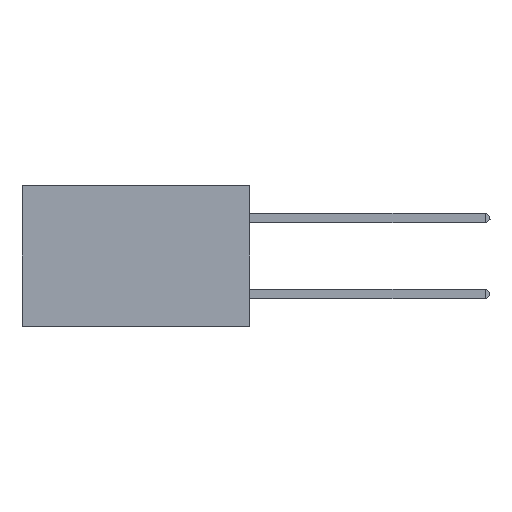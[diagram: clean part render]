
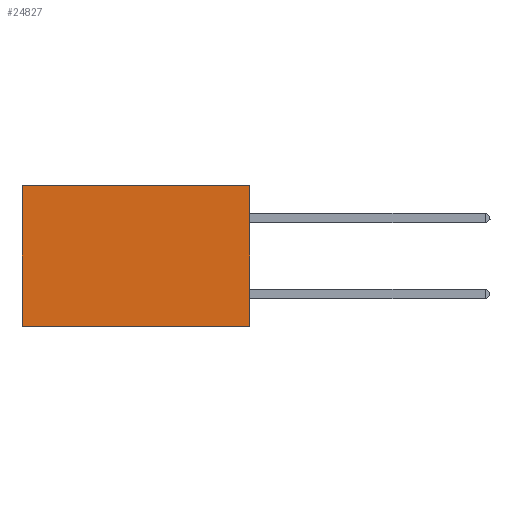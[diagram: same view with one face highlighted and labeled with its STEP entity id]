
A CAD part, left-side view. The second image highlights one B-rep face of the part: STEP entity #24827.
In plain terms, the highlighted planar face has unit normal (-1, 0, 0).
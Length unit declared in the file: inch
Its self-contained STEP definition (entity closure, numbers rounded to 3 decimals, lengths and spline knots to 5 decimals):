
#881 = CARTESIAN_POINT ( 'NONE',  ( 0.2875, 0., -0.37 ) ) ;
#1184 = EDGE_CURVE ( 'NONE', #18749, #23973, #15874, .T. ) ;
#1930 = EDGE_CURVE ( 'NONE', #21699, #4590, #20369, .T. ) ;
#2015 = LINE ( 'NONE', #881, #16713 ) ;
#2619 = CARTESIAN_POINT ( 'NONE',  ( 0.2875, 0., 0. ) ) ;
#4257 = DIRECTION ( 'NONE',  ( 0., 0., -1. ) ) ;
#4590 = VERTEX_POINT ( 'NONE', #8014 ) ;
#5044 = CARTESIAN_POINT ( 'NONE',  ( 0.2875, 0.6, 0. ) ) ;
#5109 = DIRECTION ( 'NONE',  ( 0., 0., -1. ) ) ;
#6864 = VECTOR ( 'NONE', #5109, 39.37008 ) ;
#7120 = VECTOR ( 'NONE', #7591, 39.37008 ) ;
#7141 = CARTESIAN_POINT ( 'NONE',  ( 0.2875, 0., -0.37 ) ) ;
#7591 = DIRECTION ( 'NONE',  ( 0., 1., 0. ) ) ;
#8014 = CARTESIAN_POINT ( 'NONE',  ( 0.2875, 0.6, -0.37 ) ) ;
#8030 = VECTOR ( 'NONE', #24412, 39.37008 ) ;
#9557 = AXIS2_PLACEMENT_3D ( 'NONE', #21418, #11564, #4257 ) ;
#10804 = ORIENTED_EDGE ( 'NONE', *, *, #1184, .F. ) ;
#11564 = DIRECTION ( 'NONE',  ( 1., 0., 0. ) ) ;
#11733 = ORIENTED_EDGE ( 'NONE', *, *, #13961, .F. ) ;
#12681 = FACE_OUTER_BOUND ( 'NONE', #22958, .T. ) ;
#13961 = EDGE_CURVE ( 'NONE', #23973, #4590, #2015, .T. ) ;
#15874 = LINE ( 'NONE', #24287, #6864 ) ;
#16334 = ORIENTED_EDGE ( 'NONE', *, *, #17135, .T. ) ;
#16713 = VECTOR ( 'NONE', #22237, 39.37008 ) ;
#17135 = EDGE_CURVE ( 'NONE', #18749, #21699, #24861, .T. ) ;
#18749 = VERTEX_POINT ( 'NONE', #2619 ) ;
#20369 = LINE ( 'NONE', #22331, #8030 ) ;
#21418 = CARTESIAN_POINT ( 'NONE',  ( 0.2875, 0., 0. ) ) ;
#21699 = VERTEX_POINT ( 'NONE', #5044 ) ;
#22237 = DIRECTION ( 'NONE',  ( 0., 1., 0. ) ) ;
#22331 = CARTESIAN_POINT ( 'NONE',  ( 0.2875, 0.6, 0. ) ) ;
#22958 = EDGE_LOOP ( 'NONE', ( #24066, #11733, #10804, #16334 ) ) ;
#22992 = CARTESIAN_POINT ( 'NONE',  ( 0.2875, 0., 0. ) ) ;
#23094 = PLANE ( 'NONE',  #9557 ) ;
#23973 = VERTEX_POINT ( 'NONE', #7141 ) ;
#24066 = ORIENTED_EDGE ( 'NONE', *, *, #1930, .T. ) ;
#24287 = CARTESIAN_POINT ( 'NONE',  ( 0.2875, 0., 0. ) ) ;
#24412 = DIRECTION ( 'NONE',  ( 0., 0., -1. ) ) ;
#24827 = ADVANCED_FACE ( 'NONE', ( #12681 ), #23094, .F. ) ;
#24861 = LINE ( 'NONE', #22992, #7120 ) ;
